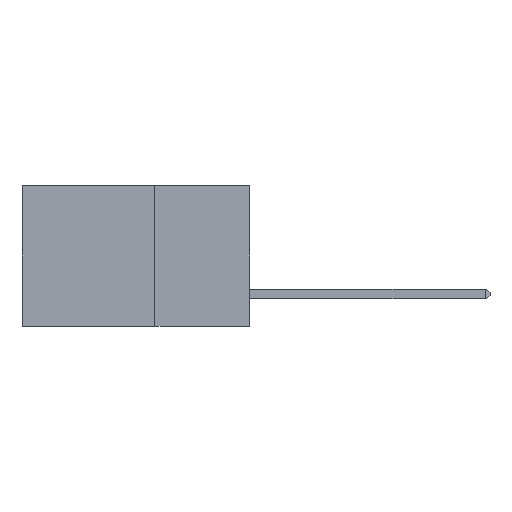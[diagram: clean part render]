
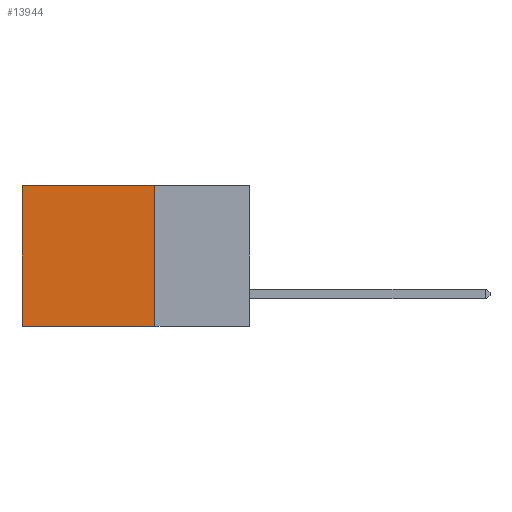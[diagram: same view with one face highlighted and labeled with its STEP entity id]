
A CAD part, left-side view. The second image highlights one B-rep face of the part: STEP entity #13944.
In plain terms, the highlighted planar face has unit normal (-1, 0, 0).
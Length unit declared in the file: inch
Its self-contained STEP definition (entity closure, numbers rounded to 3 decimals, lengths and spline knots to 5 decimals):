
#32 = LINE ( 'NONE', #17796, #18272 ) ;
#503 = VERTEX_POINT ( 'NONE', #13876 ) ;
#832 = EDGE_CURVE ( 'NONE', #17010, #4999, #17957, .T. ) ;
#2282 = EDGE_CURVE ( 'NONE', #10098, #17010, #16620, .T. ) ;
#2766 = FACE_OUTER_BOUND ( 'NONE', #9669, .T. ) ;
#2780 = AXIS2_PLACEMENT_3D ( 'NONE', #6490, #3561, #13599 ) ;
#2895 = LINE ( 'NONE', #11689, #9812 ) ;
#3291 = EDGE_CURVE ( 'NONE', #10098, #503, #32, .T. ) ;
#3561 = DIRECTION ( 'NONE',  ( 1., 0., 0. ) ) ;
#3672 = CARTESIAN_POINT ( 'NONE',  ( 0.2875, 0.25, -0.37 ) ) ;
#4374 = DIRECTION ( 'NONE',  ( 0., 1., 0. ) ) ;
#4502 = CARTESIAN_POINT ( 'NONE',  ( 0.2875, 0.6, -0.37 ) ) ;
#4999 = VERTEX_POINT ( 'NONE', #4502 ) ;
#5666 = EDGE_CURVE ( 'NONE', #503, #4999, #2895, .T. ) ;
#6375 = VECTOR ( 'NONE', #8844, 39.37008 ) ;
#6490 = CARTESIAN_POINT ( 'NONE',  ( 0.2875, 0.25, 0. ) ) ;
#8844 = DIRECTION ( 'NONE',  ( 0., 1., 0. ) ) ;
#8951 = CARTESIAN_POINT ( 'NONE',  ( 0.2875, 0.25, -0.37 ) ) ;
#9669 = EDGE_LOOP ( 'NONE', ( #17741, #17686, #17538, #17306 ) ) ;
#9812 = VECTOR ( 'NONE', #10308, 39.37008 ) ;
#10098 = VERTEX_POINT ( 'NONE', #15435 ) ;
#10308 = DIRECTION ( 'NONE',  ( 0., 0., -1. ) ) ;
#11020 = CARTESIAN_POINT ( 'NONE',  ( 0.2875, 0.25, 0. ) ) ;
#11291 = DIRECTION ( 'NONE',  ( 0., 0., -1. ) ) ;
#11689 = CARTESIAN_POINT ( 'NONE',  ( 0.2875, 0.6, 0. ) ) ;
#12219 = PLANE ( 'NONE',  #2780 ) ;
#13599 = DIRECTION ( 'NONE',  ( 0., 0., -1. ) ) ;
#13876 = CARTESIAN_POINT ( 'NONE',  ( 0.2875, 0.6, 0. ) ) ;
#13944 = ADVANCED_FACE ( 'NONE', ( #2766 ), #12219, .F. ) ;
#15435 = CARTESIAN_POINT ( 'NONE',  ( 0.2875, 0.25, 0. ) ) ;
#16191 = VECTOR ( 'NONE', #11291, 39.37008 ) ;
#16620 = LINE ( 'NONE', #11020, #16191 ) ;
#17010 = VERTEX_POINT ( 'NONE', #3672 ) ;
#17306 = ORIENTED_EDGE ( 'NONE', *, *, #3291, .T. ) ;
#17538 = ORIENTED_EDGE ( 'NONE', *, *, #2282, .F. ) ;
#17686 = ORIENTED_EDGE ( 'NONE', *, *, #832, .F. ) ;
#17741 = ORIENTED_EDGE ( 'NONE', *, *, #5666, .T. ) ;
#17796 = CARTESIAN_POINT ( 'NONE',  ( 0.2875, 0.25, 0. ) ) ;
#17957 = LINE ( 'NONE', #8951, #6375 ) ;
#18272 = VECTOR ( 'NONE', #4374, 39.37008 ) ;
